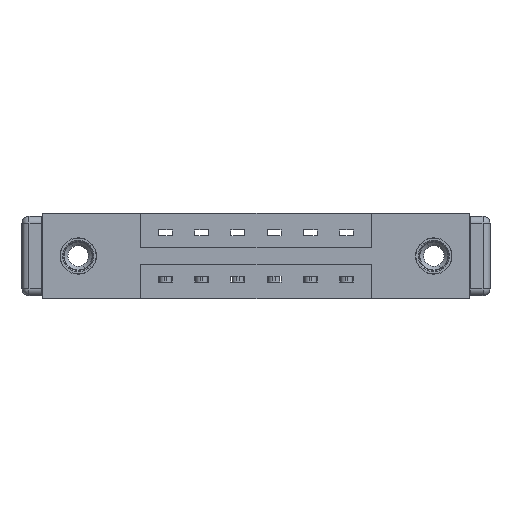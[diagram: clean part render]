
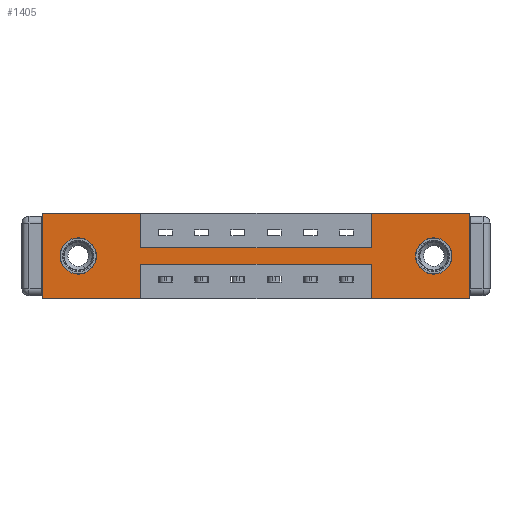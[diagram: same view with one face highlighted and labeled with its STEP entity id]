
A CAD part, front view. The second image highlights one B-rep face of the part: STEP entity #1405.
In plain terms, the highlighted planar face has unit normal (0, -1, 0).
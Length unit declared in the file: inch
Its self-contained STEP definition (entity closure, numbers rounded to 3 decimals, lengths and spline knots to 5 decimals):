
#21 = LINE ( 'NONE', #6511, #9467 ) ;
#42 = LINE ( 'NONE', #5139, #7631 ) ;
#121 = DIRECTION ( 'NONE',  ( 1., 0., 0. ) ) ;
#245 = ORIENTED_EDGE ( 'NONE', *, *, #4927, .T. ) ;
#251 = CARTESIAN_POINT ( 'NONE',  ( 0., 0., -0.37 ) ) ;
#332 = DIRECTION ( 'NONE',  ( 0., 1., 0. ) ) ;
#361 = VECTOR ( 'NONE', #5406, 39.37008 ) ;
#391 = CARTESIAN_POINT ( 'NONE',  ( 0.425, 0., -0.37 ) ) ;
#506 = VERTEX_POINT ( 'NONE', #8401 ) ;
#564 = EDGE_CURVE ( 'NONE', #10149, #10227, #10393, .T. ) ;
#586 = VERTEX_POINT ( 'NONE', #391 ) ;
#611 = DIRECTION ( 'NONE',  ( 1., 0., 0. ) ) ;
#648 = CIRCLE ( 'NONE', #6377, 0.078 ) ;
#685 = AXIS2_PLACEMENT_3D ( 'NONE', #8393, #2029, #10190 ) ;
#700 = PLANE ( 'NONE',  #2613 ) ;
#721 = CARTESIAN_POINT ( 'NONE',  ( 0., 0., -0.37 ) ) ;
#722 = CARTESIAN_POINT ( 'NONE',  ( 1.842, 0., -0.37 ) ) ;
#893 = CARTESIAN_POINT ( 'NONE',  ( 1.687, 0., -0.263 ) ) ;
#963 = EDGE_CURVE ( 'NONE', #9849, #2918, #6284, .T. ) ;
#1005 = EDGE_CURVE ( 'NONE', #5285, #1831, #5280, .T. ) ;
#1045 = LINE ( 'NONE', #5784, #6631 ) ;
#1082 = ORIENTED_EDGE ( 'NONE', *, *, #9136, .F. ) ;
#1168 = DIRECTION ( 'NONE',  ( -1., 0., 0. ) ) ;
#1207 = CIRCLE ( 'NONE', #1518, 0.078 ) ;
#1339 = DIRECTION ( 'NONE',  ( -1., 0., 0. ) ) ;
#1405 = ADVANCED_FACE ( 'NONE', ( #10396, #8286, #8136 ), #700, .T. ) ;
#1410 = VECTOR ( 'NONE', #10127, 39.37008 ) ;
#1518 = AXIS2_PLACEMENT_3D ( 'NONE', #9573, #332, #11226 ) ;
#1766 = CARTESIAN_POINT ( 'NONE',  ( 0., 0., 0. ) ) ;
#1831 = VERTEX_POINT ( 'NONE', #9485 ) ;
#2029 = DIRECTION ( 'NONE',  ( 0., 1., 0. ) ) ;
#2147 = AXIS2_PLACEMENT_3D ( 'NONE', #9269, #5551, #7502 ) ;
#2156 = DIRECTION ( 'NONE',  ( 0., 0., 1. ) ) ;
#2178 = LINE ( 'NONE', #251, #3349 ) ;
#2230 = LINE ( 'NONE', #8643, #9374 ) ;
#2385 = ORIENTED_EDGE ( 'NONE', *, *, #4922, .T. ) ;
#2601 = CARTESIAN_POINT ( 'NONE',  ( 0.425, 0., -0.15 ) ) ;
#2613 = AXIS2_PLACEMENT_3D ( 'NONE', #7146, #7941, #8034 ) ;
#2681 = VECTOR ( 'NONE', #5012, 39.37008 ) ;
#2710 = LINE ( 'NONE', #3776, #4826 ) ;
#2743 = EDGE_CURVE ( 'NONE', #2945, #9167, #1207, .T. ) ;
#2918 = VERTEX_POINT ( 'NONE', #2601 ) ;
#2945 = VERTEX_POINT ( 'NONE', #4427 ) ;
#3032 = ORIENTED_EDGE ( 'NONE', *, *, #564, .F. ) ;
#3153 = EDGE_CURVE ( 'NONE', #1831, #4569, #2710, .T. ) ;
#3349 = VECTOR ( 'NONE', #1168, 39.37008 ) ;
#3444 = ORIENTED_EDGE ( 'NONE', *, *, #3153, .F. ) ;
#3539 = ORIENTED_EDGE ( 'NONE', *, *, #2743, .T. ) ;
#3747 = VERTEX_POINT ( 'NONE', #10265 ) ;
#3776 = CARTESIAN_POINT ( 'NONE',  ( 1.842, 0., 0. ) ) ;
#3804 = EDGE_LOOP ( 'NONE', ( #3539, #2385 ) ) ;
#4008 = CARTESIAN_POINT ( 'NONE',  ( 0., 0., 0. ) ) ;
#4228 = EDGE_LOOP ( 'NONE', ( #8641, #4305, #7065, #5147, #3444, #4273, #4760, #4718, #7505, #8326, #3032, #1082 ) ) ;
#4252 = VECTOR ( 'NONE', #8421, 39.37008 ) ;
#4273 = ORIENTED_EDGE ( 'NONE', *, *, #1005, .F. ) ;
#4305 = ORIENTED_EDGE ( 'NONE', *, *, #7446, .F. ) ;
#4402 = VERTEX_POINT ( 'NONE', #6960 ) ;
#4427 = CARTESIAN_POINT ( 'NONE',  ( 0.155, 0., -0.107 ) ) ;
#4569 = VERTEX_POINT ( 'NONE', #722 ) ;
#4671 = LINE ( 'NONE', #6930, #2681 ) ;
#4718 = ORIENTED_EDGE ( 'NONE', *, *, #8612, .F. ) ;
#4760 = ORIENTED_EDGE ( 'NONE', *, *, #7174, .F. ) ;
#4826 = VECTOR ( 'NONE', #7603, 39.37008 ) ;
#4872 = CARTESIAN_POINT ( 'NONE',  ( 0.425, 0., 0. ) ) ;
#4922 = EDGE_CURVE ( 'NONE', #9167, #2945, #5005, .T. ) ;
#4927 = EDGE_CURVE ( 'NONE', #9442, #6320, #7161, .T. ) ;
#5005 = CIRCLE ( 'NONE', #2147, 0.078 ) ;
#5012 = DIRECTION ( 'NONE',  ( 0., 0., 1. ) ) ;
#5079 = CARTESIAN_POINT ( 'NONE',  ( 1.417, 0., -0.15 ) ) ;
#5139 = CARTESIAN_POINT ( 'NONE',  ( 0.425, 0., -0.15 ) ) ;
#5147 = ORIENTED_EDGE ( 'NONE', *, *, #8402, .F. ) ;
#5280 = LINE ( 'NONE', #11079, #1410 ) ;
#5285 = VERTEX_POINT ( 'NONE', #8269 ) ;
#5406 = DIRECTION ( 'NONE',  ( -1., 0., 0. ) ) ;
#5551 = DIRECTION ( 'NONE',  ( 0., 1., 0. ) ) ;
#5784 = CARTESIAN_POINT ( 'NONE',  ( 0., 0., -0.37 ) ) ;
#6284 = LINE ( 'NONE', #7337, #10548 ) ;
#6320 = VERTEX_POINT ( 'NONE', #893 ) ;
#6377 = AXIS2_PLACEMENT_3D ( 'NONE', #8095, #11738, #8247 ) ;
#6511 = CARTESIAN_POINT ( 'NONE',  ( 0., 0., 0. ) ) ;
#6631 = VECTOR ( 'NONE', #1339, 39.37008 ) ;
#6677 = EDGE_LOOP ( 'NONE', ( #245, #11520 ) ) ;
#6687 = CARTESIAN_POINT ( 'NONE',  ( 1.417, 0., -0.37 ) ) ;
#6930 = CARTESIAN_POINT ( 'NONE',  ( 1.417, 0., 0. ) ) ;
#6960 = CARTESIAN_POINT ( 'NONE',  ( 1.417, 0., -0.22 ) ) ;
#7056 = EDGE_CURVE ( 'NONE', #506, #4402, #10514, .T. ) ;
#7065 = ORIENTED_EDGE ( 'NONE', *, *, #7056, .F. ) ;
#7146 = CARTESIAN_POINT ( 'NONE',  ( 0., 0., -0.37 ) ) ;
#7161 = CIRCLE ( 'NONE', #685, 0.078 ) ;
#7174 = EDGE_CURVE ( 'NONE', #9312, #5285, #4671, .T. ) ;
#7337 = CARTESIAN_POINT ( 'NONE',  ( 0.425, 0., 0. ) ) ;
#7363 = EDGE_CURVE ( 'NONE', #6320, #9442, #648, .T. ) ;
#7446 = EDGE_CURVE ( 'NONE', #4402, #3747, #8383, .T. ) ;
#7502 = DIRECTION ( 'NONE',  ( 0., 0., 1. ) ) ;
#7505 = ORIENTED_EDGE ( 'NONE', *, *, #963, .F. ) ;
#7575 = CARTESIAN_POINT ( 'NONE',  ( 0.155, 0., -0.263 ) ) ;
#7603 = DIRECTION ( 'NONE',  ( 0., 0., -1. ) ) ;
#7631 = VECTOR ( 'NONE', #611, 39.37008 ) ;
#7941 = DIRECTION ( 'NONE',  ( 0., -1., 0. ) ) ;
#8034 = DIRECTION ( 'NONE',  ( 0., 0., -1. ) ) ;
#8095 = CARTESIAN_POINT ( 'NONE',  ( 1.687, 0., -0.185 ) ) ;
#8136 = FACE_OUTER_BOUND ( 'NONE', #4228, .T. ) ;
#8247 = DIRECTION ( 'NONE',  ( 0., 0., -1. ) ) ;
#8269 = CARTESIAN_POINT ( 'NONE',  ( 1.417, 0., 0. ) ) ;
#8286 = FACE_BOUND ( 'NONE', #3804, .T. ) ;
#8326 = ORIENTED_EDGE ( 'NONE', *, *, #9610, .F. ) ;
#8383 = LINE ( 'NONE', #9055, #361 ) ;
#8393 = CARTESIAN_POINT ( 'NONE',  ( 1.687, 0., -0.185 ) ) ;
#8401 = CARTESIAN_POINT ( 'NONE',  ( 1.417, 0., -0.37 ) ) ;
#8402 = EDGE_CURVE ( 'NONE', #4569, #506, #1045, .T. ) ;
#8421 = DIRECTION ( 'NONE',  ( 0., 0., 1. ) ) ;
#8612 = EDGE_CURVE ( 'NONE', #2918, #9312, #42, .T. ) ;
#8641 = ORIENTED_EDGE ( 'NONE', *, *, #11803, .F. ) ;
#8643 = CARTESIAN_POINT ( 'NONE',  ( 0.425, 0., -0.37 ) ) ;
#9055 = CARTESIAN_POINT ( 'NONE',  ( 0.425, 0., -0.22 ) ) ;
#9132 = VECTOR ( 'NONE', #2156, 39.37008 ) ;
#9136 = EDGE_CURVE ( 'NONE', #586, #10149, #2178, .T. ) ;
#9167 = VERTEX_POINT ( 'NONE', #7575 ) ;
#9269 = CARTESIAN_POINT ( 'NONE',  ( 0.155, 0., -0.185 ) ) ;
#9312 = VERTEX_POINT ( 'NONE', #5079 ) ;
#9374 = VECTOR ( 'NONE', #10494, 39.37008 ) ;
#9442 = VERTEX_POINT ( 'NONE', #10591 ) ;
#9467 = VECTOR ( 'NONE', #121, 39.37008 ) ;
#9485 = CARTESIAN_POINT ( 'NONE',  ( 1.842, 0., 0. ) ) ;
#9573 = CARTESIAN_POINT ( 'NONE',  ( 0.155, 0., -0.185 ) ) ;
#9610 = EDGE_CURVE ( 'NONE', #10227, #9849, #21, .T. ) ;
#9849 = VERTEX_POINT ( 'NONE', #4872 ) ;
#10127 = DIRECTION ( 'NONE',  ( 1., 0., 0. ) ) ;
#10149 = VERTEX_POINT ( 'NONE', #721 ) ;
#10190 = DIRECTION ( 'NONE',  ( 0., 0., -1. ) ) ;
#10227 = VERTEX_POINT ( 'NONE', #1766 ) ;
#10265 = CARTESIAN_POINT ( 'NONE',  ( 0.425, 0., -0.22 ) ) ;
#10393 = LINE ( 'NONE', #4008, #9132 ) ;
#10396 = FACE_BOUND ( 'NONE', #6677, .T. ) ;
#10494 = DIRECTION ( 'NONE',  ( 0., 0., -1. ) ) ;
#10514 = LINE ( 'NONE', #6687, #4252 ) ;
#10548 = VECTOR ( 'NONE', #10924, 39.37008 ) ;
#10591 = CARTESIAN_POINT ( 'NONE',  ( 1.687, 0., -0.107 ) ) ;
#10924 = DIRECTION ( 'NONE',  ( 0., 0., -1. ) ) ;
#11079 = CARTESIAN_POINT ( 'NONE',  ( 0., 0., 0. ) ) ;
#11226 = DIRECTION ( 'NONE',  ( 0., 0., 1. ) ) ;
#11520 = ORIENTED_EDGE ( 'NONE', *, *, #7363, .T. ) ;
#11738 = DIRECTION ( 'NONE',  ( 0., 1., 0. ) ) ;
#11803 = EDGE_CURVE ( 'NONE', #3747, #586, #2230, .T. ) ;
